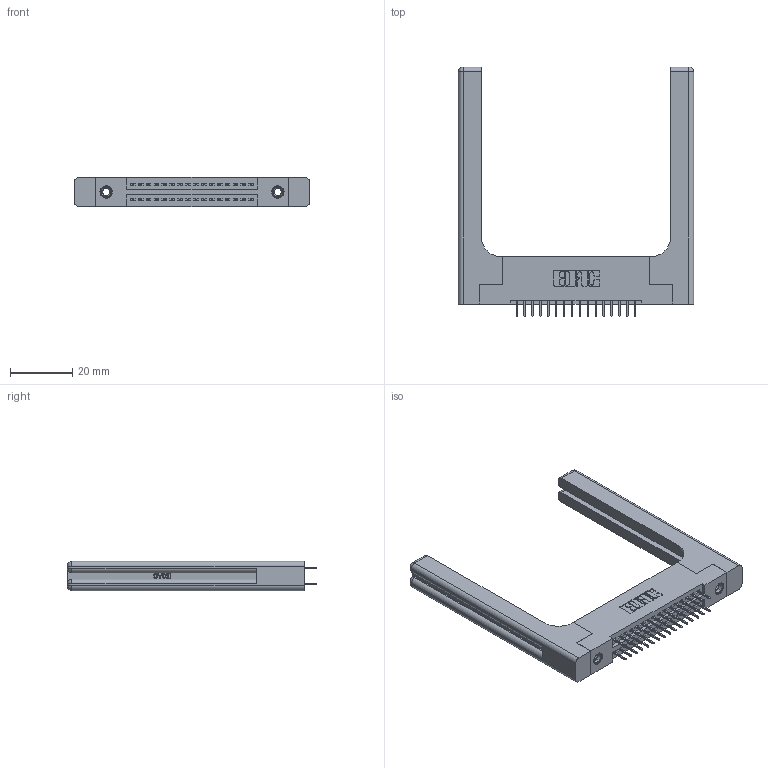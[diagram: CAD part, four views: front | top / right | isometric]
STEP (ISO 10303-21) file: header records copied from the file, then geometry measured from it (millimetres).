
FILE_DESCRIPTION (( 'STEP AP203' ), '1' );
FILE_NAME ('395-032-524-258.STEP', '2019-10-17T15:44:52', ( '' ), ( '' ), 'SwSTEP 2.0', 'SolidWorks 2016', '' );
FILE_SCHEMA (( 'CONFIG_CONTROL_DESIGN' ));
Length unit declared in the file: inch
Products named in the file (5): 395-032-524-258; 345 Part_Flush Mounting Lugs - 0.156 Dia-TH; 345-292-001_345-293-124; 345-250-001_345-250-001-102; 345-220-058_345-220-058
Assembly tree (37 placements, depth 2):
  395-032-524-258
    345 Part_Flush Mounting Lugs - 0.156 Dia-TH
    345-292-001_345-293-124  x32
    345-250-001_345-250-001-102  x2
    345-220-058_345-220-058  x2
Bounding box: 75.67 x 80.31 x 9.4 mm (x, y, z)
Volume: 15535.7 mm3; surface area: 14864.2 mm2
Topology: 37 solids, 37 shells, 2110 faces, 5903 edges, 3786 vertices
Faces by surface type: plane 1476, cylinder 574, bspline 36, cone 12, sphere 8, torus 4
Entity records: 21310 total; most frequent: CARTESIAN_POINT 4589, ORIENTED_EDGE 3320, DIRECTION 3012, EDGE_CURVE 1660, VECTOR 1376, LINE 1376, VERTEX_POINT 1094, AXIS2_PLACEMENT_3D 818
